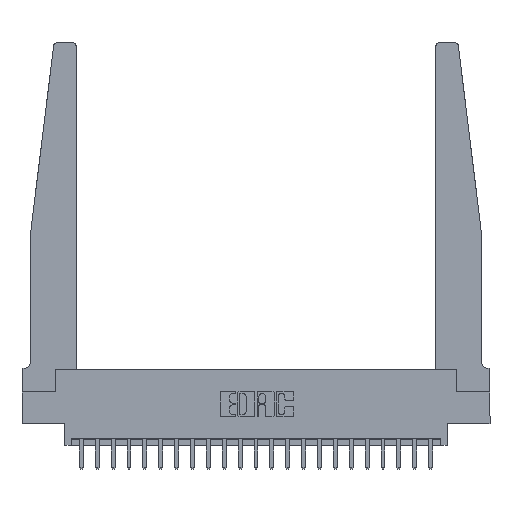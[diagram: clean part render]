
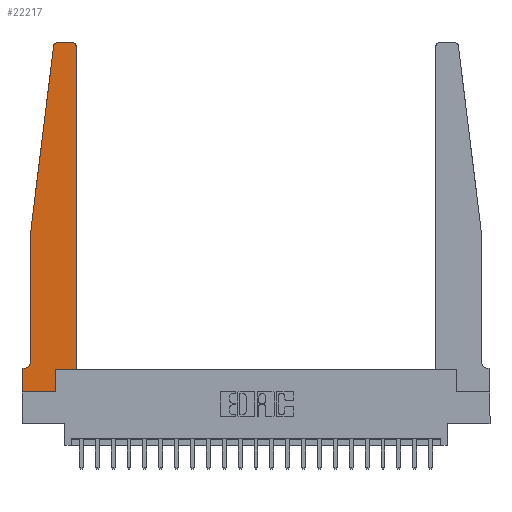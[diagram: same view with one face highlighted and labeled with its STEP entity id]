
A CAD part, top view. The second image highlights one B-rep face of the part: STEP entity #22217.
In plain terms, the highlighted planar face has unit normal (0, 0, 1).
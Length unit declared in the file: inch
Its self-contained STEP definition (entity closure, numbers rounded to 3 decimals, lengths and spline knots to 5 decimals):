
#51 = VERTEX_POINT ( 'NONE', #19634 ) ;
#664 = LINE ( 'NONE', #10077, #4358 ) ;
#698 = DIRECTION ( 'NONE',  ( 0., 1., 0. ) ) ;
#930 = VECTOR ( 'NONE', #8499, 39.37008 ) ;
#951 = DIRECTION ( 'NONE',  ( 1., 0., 0. ) ) ;
#1283 = CARTESIAN_POINT ( 'NONE',  ( 0.27653, 2.72, 0.37 ) ) ;
#1348 = DIRECTION ( 'NONE',  ( 0., 1., 0. ) ) ;
#2109 = VERTEX_POINT ( 'NONE', #10820 ) ;
#3097 = EDGE_CURVE ( 'NONE', #18913, #51, #11639, .T. ) ;
#3112 = DIRECTION ( 'NONE',  ( 1., 0., 0. ) ) ;
#3359 = VECTOR ( 'NONE', #19264, 39.37008 ) ;
#3505 = VERTEX_POINT ( 'NONE', #3628 ) ;
#3628 = CARTESIAN_POINT ( 'NONE',  ( 0.425, 0.18, 0.37 ) ) ;
#3861 = VECTOR ( 'NONE', #698, 39.37008 ) ;
#4358 = VECTOR ( 'NONE', #15292, 39.37008 ) ;
#4457 = AXIS2_PLACEMENT_3D ( 'NONE', #18837, #8444, #20512 ) ;
#4510 = VERTEX_POINT ( 'NONE', #12087 ) ;
#4818 = AXIS2_PLACEMENT_3D ( 'NONE', #1283, #13699, #3112 ) ;
#4952 = CARTESIAN_POINT ( 'NONE',  ( 0.425, 2.72, 0.37 ) ) ;
#4983 = CARTESIAN_POINT ( 'NONE',  ( 0.2605, 0.18, 0.37 ) ) ;
#5138 = CARTESIAN_POINT ( 'NONE',  ( 0., 0., 0.37 ) ) ;
#5187 = VECTOR ( 'NONE', #1348, 39.37008 ) ;
#5189 = VERTEX_POINT ( 'NONE', #12280 ) ;
#5746 = LINE ( 'NONE', #15409, #930 ) ;
#5824 = VECTOR ( 'NONE', #8254, 39.37008 ) ;
#6131 = EDGE_CURVE ( 'NONE', #18912, #2109, #5746, .T. ) ;
#6172 = EDGE_CURVE ( 'NONE', #3505, #13106, #19101, .T. ) ;
#6212 = VERTEX_POINT ( 'NONE', #12145 ) ;
#6398 = LINE ( 'NONE', #6494, #5824 ) ;
#6494 = CARTESIAN_POINT ( 'NONE',  ( 0.065, 0.1875, 0.37 ) ) ;
#7091 = DIRECTION ( 'NONE',  ( 0., -1., 0. ) ) ;
#7118 = CARTESIAN_POINT ( 'NONE',  ( 0., 0., 0.37 ) ) ;
#7164 = ORIENTED_EDGE ( 'NONE', *, *, #14981, .T. ) ;
#7235 = ORIENTED_EDGE ( 'NONE', *, *, #10525, .T. ) ;
#7270 = CIRCLE ( 'NONE', #4818, 0.03 ) ;
#7329 = LINE ( 'NONE', #19824, #11416 ) ;
#7388 = CARTESIAN_POINT ( 'NONE',  ( 0.015, 0.2375, 0.37 ) ) ;
#7494 = ORIENTED_EDGE ( 'NONE', *, *, #19109, .T. ) ;
#8111 = PLANE ( 'NONE',  #16093 ) ;
#8120 = VECTOR ( 'NONE', #7091, 39.37008 ) ;
#8254 = DIRECTION ( 'NONE',  ( -1., 0., 0. ) ) ;
#8444 = DIRECTION ( 'NONE',  ( 0., 0., 1. ) ) ;
#8499 = DIRECTION ( 'NONE',  ( -0.122, -0.992, 0. ) ) ;
#9027 = VERTEX_POINT ( 'NONE', #4983 ) ;
#9087 = VERTEX_POINT ( 'NONE', #5138 ) ;
#9142 = DIRECTION ( 'NONE',  ( -1., 0., 0. ) ) ;
#9459 = CARTESIAN_POINT ( 'NONE',  ( 0.395, 2.75, 0.37 ) ) ;
#9659 = ORIENTED_EDGE ( 'NONE', *, *, #3097, .T. ) ;
#9884 = CARTESIAN_POINT ( 'NONE',  ( 0.065, 0.2375, 0.37 ) ) ;
#10077 = CARTESIAN_POINT ( 'NONE',  ( 0.425, 0.18, 0.37 ) ) ;
#10294 = ORIENTED_EDGE ( 'NONE', *, *, #6131, .T. ) ;
#10525 = EDGE_CURVE ( 'NONE', #5189, #9027, #21260, .T. ) ;
#10820 = CARTESIAN_POINT ( 'NONE',  ( 0.065, 1.25, 0.37 ) ) ;
#10978 = ORIENTED_EDGE ( 'NONE', *, *, #18184, .T. ) ;
#11154 = ORIENTED_EDGE ( 'NONE', *, *, #21722, .T. ) ;
#11303 = DIRECTION ( 'NONE',  ( 0., -1., 0. ) ) ;
#11322 = ORIENTED_EDGE ( 'NONE', *, *, #12709, .T. ) ;
#11416 = VECTOR ( 'NONE', #11303, 39.37008 ) ;
#11598 = DIRECTION ( 'NONE',  ( 0., 0., 1. ) ) ;
#11639 = LINE ( 'NONE', #16608, #20265 ) ;
#11796 = ORIENTED_EDGE ( 'NONE', *, *, #20317, .T. ) ;
#12087 = CARTESIAN_POINT ( 'NONE',  ( 0.015, 0.1875, 0.37 ) ) ;
#12103 = ORIENTED_EDGE ( 'NONE', *, *, #18681, .T. ) ;
#12128 = ORIENTED_EDGE ( 'NONE', *, *, #14165, .T. ) ;
#12145 = CARTESIAN_POINT ( 'NONE',  ( 0., 0.1875, 0.37 ) ) ;
#12280 = CARTESIAN_POINT ( 'NONE',  ( 0.2605, 0., 0.37 ) ) ;
#12698 = EDGE_LOOP ( 'NONE', ( #9659, #11154, #10294, #11796, #11322, #12128, #12103, #10978, #7235, #7164, #19489, #7494 ) ) ;
#12709 = EDGE_CURVE ( 'NONE', #20426, #4510, #20680, .T. ) ;
#12748 = LINE ( 'NONE', #15732, #8120 ) ;
#13106 = VERTEX_POINT ( 'NONE', #4952 ) ;
#13153 = CARTESIAN_POINT ( 'NONE',  ( 0.2605, 0.18, 0.37 ) ) ;
#13699 = DIRECTION ( 'NONE',  ( 0., 0., 1. ) ) ;
#14165 = EDGE_CURVE ( 'NONE', #4510, #6212, #6398, .T. ) ;
#14981 = EDGE_CURVE ( 'NONE', #9027, #3505, #664, .T. ) ;
#15292 = DIRECTION ( 'NONE',  ( 1., 0., 0. ) ) ;
#15409 = CARTESIAN_POINT ( 'NONE',  ( 0.065, 1.25, 0.37 ) ) ;
#15685 = FACE_OUTER_BOUND ( 'NONE', #12698, .T. ) ;
#15732 = CARTESIAN_POINT ( 'NONE',  ( 0., 0., 0.37 ) ) ;
#16093 = AXIS2_PLACEMENT_3D ( 'NONE', #20187, #11598, #951 ) ;
#16608 = CARTESIAN_POINT ( 'NONE',  ( 0.25, 2.75, 0.37 ) ) ;
#17228 = CARTESIAN_POINT ( 'NONE',  ( 0.425, 0.18, 0.37 ) ) ;
#18184 = EDGE_CURVE ( 'NONE', #9087, #5189, #21329, .T. ) ;
#18363 = DIRECTION ( 'NONE',  ( -1., 0., 0. ) ) ;
#18681 = EDGE_CURVE ( 'NONE', #6212, #9087, #12748, .T. ) ;
#18837 = CARTESIAN_POINT ( 'NONE',  ( 0.395, 2.72, 0.37 ) ) ;
#18912 = VERTEX_POINT ( 'NONE', #19794 ) ;
#18913 = VERTEX_POINT ( 'NONE', #9459 ) ;
#19025 = AXIS2_PLACEMENT_3D ( 'NONE', #7388, #19509, #9142 ) ;
#19101 = LINE ( 'NONE', #17228, #5187 ) ;
#19109 = EDGE_CURVE ( 'NONE', #13106, #18913, #22345, .T. ) ;
#19264 = DIRECTION ( 'NONE',  ( 1., 0., 0. ) ) ;
#19489 = ORIENTED_EDGE ( 'NONE', *, *, #6172, .T. ) ;
#19509 = DIRECTION ( 'NONE',  ( 0., 0., -1. ) ) ;
#19634 = CARTESIAN_POINT ( 'NONE',  ( 0.27653, 2.75, 0.37 ) ) ;
#19794 = CARTESIAN_POINT ( 'NONE',  ( 0.24675, 2.72367, 0.37 ) ) ;
#19824 = CARTESIAN_POINT ( 'NONE',  ( 0.065, 1.25, 0.37 ) ) ;
#20187 = CARTESIAN_POINT ( 'NONE',  ( 0., 0.1875, 0.37 ) ) ;
#20265 = VECTOR ( 'NONE', #18363, 39.37008 ) ;
#20317 = EDGE_CURVE ( 'NONE', #2109, #20426, #7329, .T. ) ;
#20426 = VERTEX_POINT ( 'NONE', #9884 ) ;
#20512 = DIRECTION ( 'NONE',  ( 1., 0., 0. ) ) ;
#20680 = CIRCLE ( 'NONE', #19025, 0.05 ) ;
#21260 = LINE ( 'NONE', #13153, #3861 ) ;
#21329 = LINE ( 'NONE', #7118, #3359 ) ;
#21722 = EDGE_CURVE ( 'NONE', #51, #18912, #7270, .T. ) ;
#22217 = ADVANCED_FACE ( 'NONE', ( #15685 ), #8111, .T. ) ;
#22345 = CIRCLE ( 'NONE', #4457, 0.03 ) ;
